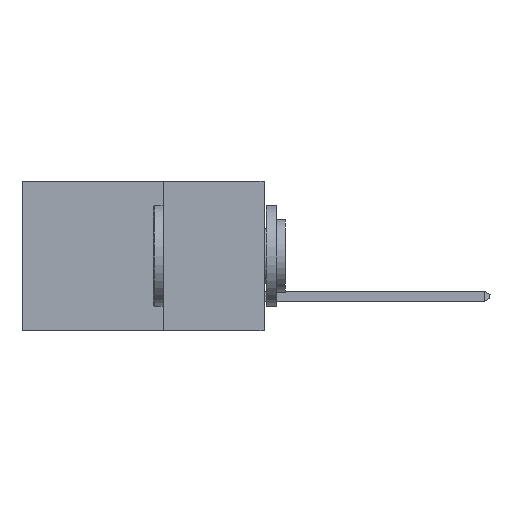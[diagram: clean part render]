
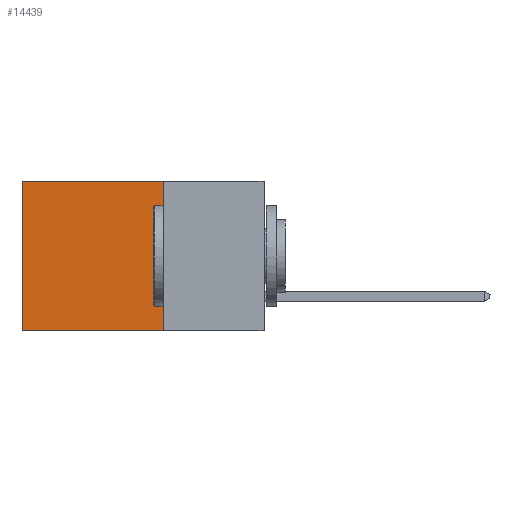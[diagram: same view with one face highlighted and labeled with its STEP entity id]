
A CAD part, left-side view. The second image highlights one B-rep face of the part: STEP entity #14439.
In plain terms, the highlighted planar face has unit normal (-1, 0, 0).
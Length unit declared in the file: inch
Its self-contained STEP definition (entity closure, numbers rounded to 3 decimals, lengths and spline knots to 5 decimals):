
#482 = LINE ( 'NONE', #6098, #15527 ) ;
#1943 = VERTEX_POINT ( 'NONE', #3720 ) ;
#3720 = CARTESIAN_POINT ( 'NONE',  ( 0.2615, 0.6, 0. ) ) ;
#4789 = LINE ( 'NONE', #7749, #5963 ) ;
#4796 = CARTESIAN_POINT ( 'NONE',  ( 0.2615, 0.6, -0.37 ) ) ;
#4961 = CARTESIAN_POINT ( 'NONE',  ( 0.2615, 0.25, 0. ) ) ;
#5067 = VERTEX_POINT ( 'NONE', #7779 ) ;
#5071 = LINE ( 'NONE', #9318, #5866 ) ;
#5382 = EDGE_CURVE ( 'NONE', #1943, #6830, #4789, .T. ) ;
#5866 = VECTOR ( 'NONE', #14881, 39.37008 ) ;
#5963 = VECTOR ( 'NONE', #10514, 39.37008 ) ;
#5974 = DIRECTION ( 'NONE',  ( 0., 0., -1. ) ) ;
#6035 = VERTEX_POINT ( 'NONE', #4961 ) ;
#6098 = CARTESIAN_POINT ( 'NONE',  ( 0.2615, 0.25, 0. ) ) ;
#6830 = VERTEX_POINT ( 'NONE', #4796 ) ;
#7630 = CARTESIAN_POINT ( 'NONE',  ( 0.2615, 0.25, -0.37 ) ) ;
#7749 = CARTESIAN_POINT ( 'NONE',  ( 0.2615, 0.6, -0.37 ) ) ;
#7779 = CARTESIAN_POINT ( 'NONE',  ( 0.2615, 0.25, -0.37 ) ) ;
#8631 = DIRECTION ( 'NONE',  ( 0., 0., -1. ) ) ;
#8750 = ORIENTED_EDGE ( 'NONE', *, *, #5382, .T. ) ;
#9318 = CARTESIAN_POINT ( 'NONE',  ( 0.2615, 0.25, -0.37 ) ) ;
#9650 = CARTESIAN_POINT ( 'NONE',  ( 0.2615, 0.25, -0.37 ) ) ;
#9940 = FACE_OUTER_BOUND ( 'NONE', #12311, .T. ) ;
#10002 = LINE ( 'NONE', #9650, #11389 ) ;
#10514 = DIRECTION ( 'NONE',  ( 0., 0., -1. ) ) ;
#10519 = ORIENTED_EDGE ( 'NONE', *, *, #13521, .F. ) ;
#11389 = VECTOR ( 'NONE', #8631, 39.37008 ) ;
#11711 = DIRECTION ( 'NONE',  ( 0., 1., 0. ) ) ;
#11932 = DIRECTION ( 'NONE',  ( 1., 0., 0. ) ) ;
#12311 = EDGE_LOOP ( 'NONE', ( #8750, #14464, #10519, #18086 ) ) ;
#13203 = PLANE ( 'NONE',  #15480 ) ;
#13521 = EDGE_CURVE ( 'NONE', #6035, #5067, #10002, .T. ) ;
#14439 = ADVANCED_FACE ( 'NONE', ( #9940 ), #13203, .F. ) ;
#14464 = ORIENTED_EDGE ( 'NONE', *, *, #16248, .F. ) ;
#14881 = DIRECTION ( 'NONE',  ( 0., 1., 0. ) ) ;
#15480 = AXIS2_PLACEMENT_3D ( 'NONE', #7630, #11932, #5974 ) ;
#15527 = VECTOR ( 'NONE', #11711, 39.37008 ) ;
#16148 = EDGE_CURVE ( 'NONE', #6035, #1943, #482, .T. ) ;
#16248 = EDGE_CURVE ( 'NONE', #5067, #6830, #5071, .T. ) ;
#18086 = ORIENTED_EDGE ( 'NONE', *, *, #16148, .T. ) ;
